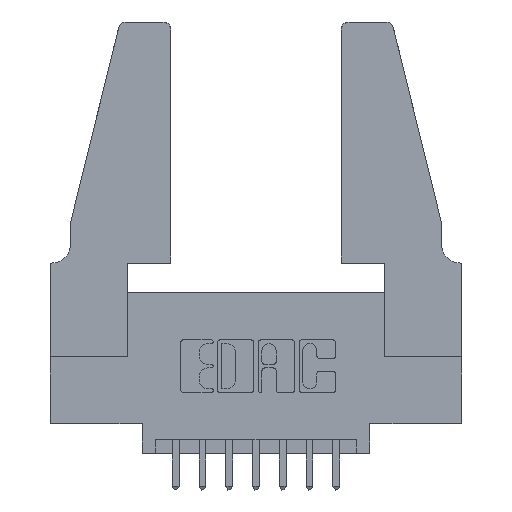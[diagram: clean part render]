
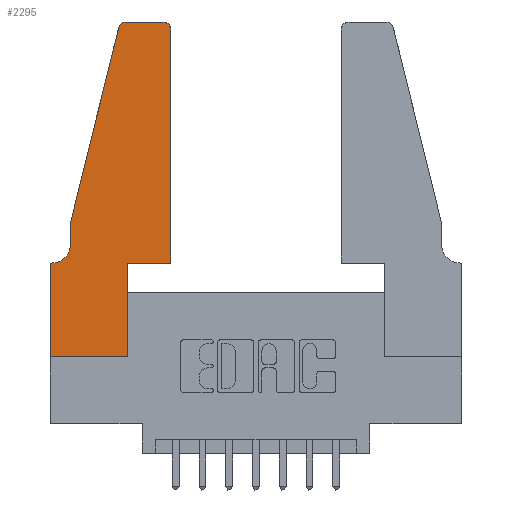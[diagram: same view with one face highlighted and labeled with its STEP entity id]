
A CAD part, top view. The second image highlights one B-rep face of the part: STEP entity #2295.
In plain terms, the highlighted planar face has unit normal (0, 0, 1).
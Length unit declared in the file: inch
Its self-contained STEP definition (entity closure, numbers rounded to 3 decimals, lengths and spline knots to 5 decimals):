
#74 = LINE ( 'NONE', #11500, #10061 ) ;
#209 = AXIS2_PLACEMENT_3D ( 'NONE', #2122, #8874, #3090 ) ;
#328 = CARTESIAN_POINT ( 'NONE',  ( 0.4505, 0.35, 0.37 ) ) ;
#382 = EDGE_CURVE ( 'NONE', #6844, #2311, #5477, .T. ) ;
#401 = VERTEX_POINT ( 'NONE', #3367 ) ;
#485 = CARTESIAN_POINT ( 'NONE',  ( 0.0755, 0.5, 0.37 ) ) ;
#541 = LINE ( 'NONE', #10446, #2849 ) ;
#887 = DIRECTION ( 'NONE',  ( 0., -1., 0. ) ) ;
#928 = EDGE_CURVE ( 'NONE', #4702, #10897, #2279, .T. ) ;
#1091 = DIRECTION ( 'NONE',  ( -0.239, -0.971, 0. ) ) ;
#1434 = EDGE_CURVE ( 'NONE', #10897, #5104, #6479, .T. ) ;
#1604 = VERTEX_POINT ( 'NONE', #1941 ) ;
#1919 = DIRECTION ( 'NONE',  ( 0., 1., 0. ) ) ;
#1941 = CARTESIAN_POINT ( 'NONE',  ( 0.2865, 0., 0.37 ) ) ;
#1979 = ORIENTED_EDGE ( 'NONE', *, *, #10025, .T. ) ;
#2013 = CARTESIAN_POINT ( 'NONE',  ( 0.0755, 0.42, 0.37 ) ) ;
#2122 = CARTESIAN_POINT ( 'NONE',  ( 0.0055, 0.42, 0.37 ) ) ;
#2279 = CIRCLE ( 'NONE', #3475, 0.03 ) ;
#2295 = ADVANCED_FACE ( 'NONE', ( #2711 ), #9443, .T. ) ;
#2311 = VERTEX_POINT ( 'NONE', #5641 ) ;
#2376 = EDGE_LOOP ( 'NONE', ( #1979, #10501, #11149, #3997, #9393, #7871, #9569, #4643, #2788, #7935, #9923, #3000 ) ) ;
#2415 = VECTOR ( 'NONE', #887, 39.37008 ) ;
#2492 = VERTEX_POINT ( 'NONE', #2013 ) ;
#2711 = FACE_OUTER_BOUND ( 'NONE', #2376, .T. ) ;
#2788 = ORIENTED_EDGE ( 'NONE', *, *, #5340, .T. ) ;
#2849 = VECTOR ( 'NONE', #3736, 39.37008 ) ;
#3000 = ORIENTED_EDGE ( 'NONE', *, *, #10651, .T. ) ;
#3090 = DIRECTION ( 'NONE',  ( -1., 0., 0. ) ) ;
#3192 = EDGE_CURVE ( 'NONE', #2311, #6945, #9752, .T. ) ;
#3367 = CARTESIAN_POINT ( 'NONE',  ( 0., 0., 0.37 ) ) ;
#3411 = CARTESIAN_POINT ( 'NONE',  ( 0.4505, 1.22, 0.37 ) ) ;
#3475 = AXIS2_PLACEMENT_3D ( 'NONE', #4786, #5442, #5460 ) ;
#3736 = DIRECTION ( 'NONE',  ( -1., 0., 0. ) ) ;
#3936 = VECTOR ( 'NONE', #1091, 39.37008 ) ;
#3997 = ORIENTED_EDGE ( 'NONE', *, *, #9315, .T. ) ;
#3998 = VECTOR ( 'NONE', #5031, 39.37008 ) ;
#4186 = LINE ( 'NONE', #8678, #9007 ) ;
#4343 = VERTEX_POINT ( 'NONE', #10725 ) ;
#4475 = DIRECTION ( 'NONE',  ( 1., 0., 0. ) ) ;
#4520 = LINE ( 'NONE', #11569, #9329 ) ;
#4643 = ORIENTED_EDGE ( 'NONE', *, *, #11556, .T. ) ;
#4702 = VERTEX_POINT ( 'NONE', #11522 ) ;
#4786 = CARTESIAN_POINT ( 'NONE',  ( 0.284, 1.22, 0.37 ) ) ;
#4874 = DIRECTION ( 'NONE',  ( -1., 0., 0. ) ) ;
#4983 = LINE ( 'NONE', #8634, #2415 ) ;
#5031 = DIRECTION ( 'NONE',  ( 1., 0., 0. ) ) ;
#5104 = VERTEX_POINT ( 'NONE', #9314 ) ;
#5340 = EDGE_CURVE ( 'NONE', #1604, #6844, #4186, .T. ) ;
#5442 = DIRECTION ( 'NONE',  ( 0., 0., 1. ) ) ;
#5460 = DIRECTION ( 'NONE',  ( 1., 0., 0. ) ) ;
#5477 = LINE ( 'NONE', #328, #10252 ) ;
#5494 = CARTESIAN_POINT ( 'NONE',  ( 0.4205, 1.22, 0.37 ) ) ;
#5641 = CARTESIAN_POINT ( 'NONE',  ( 0.4505, 0.35, 0.37 ) ) ;
#5959 = VERTEX_POINT ( 'NONE', #10536 ) ;
#5960 = CARTESIAN_POINT ( 'NONE',  ( 0., 0., 0.37 ) ) ;
#6087 = EDGE_CURVE ( 'NONE', #2492, #5959, #6267, .T. ) ;
#6267 = CIRCLE ( 'NONE', #209, 0.07 ) ;
#6432 = DIRECTION ( 'NONE',  ( 1., 0., 0. ) ) ;
#6479 = LINE ( 'NONE', #485, #3936 ) ;
#6728 = DIRECTION ( 'NONE',  ( 0., -1., 0. ) ) ;
#6844 = VERTEX_POINT ( 'NONE', #10929 ) ;
#6845 = LINE ( 'NONE', #5960, #3998 ) ;
#6945 = VERTEX_POINT ( 'NONE', #3411 ) ;
#7037 = CARTESIAN_POINT ( 'NONE',  ( 0.4505, 0.35, 0.37 ) ) ;
#7193 = VECTOR ( 'NONE', #12448, 39.37008 ) ;
#7871 = ORIENTED_EDGE ( 'NONE', *, *, #9899, .T. ) ;
#7935 = ORIENTED_EDGE ( 'NONE', *, *, #382, .T. ) ;
#8634 = CARTESIAN_POINT ( 'NONE',  ( 0.0755, 0.5, 0.37 ) ) ;
#8678 = CARTESIAN_POINT ( 'NONE',  ( 0.2865, 0.35, 0.37 ) ) ;
#8770 = VERTEX_POINT ( 'NONE', #9722 ) ;
#8874 = DIRECTION ( 'NONE',  ( 0., 0., -1. ) ) ;
#9007 = VECTOR ( 'NONE', #1919, 39.37008 ) ;
#9314 = CARTESIAN_POINT ( 'NONE',  ( 0.0755, 0.5, 0.37 ) ) ;
#9315 = EDGE_CURVE ( 'NONE', #5104, #2492, #4983, .T. ) ;
#9329 = VECTOR ( 'NONE', #4874, 39.37008 ) ;
#9393 = ORIENTED_EDGE ( 'NONE', *, *, #6087, .T. ) ;
#9443 = PLANE ( 'NONE',  #11101 ) ;
#9569 = ORIENTED_EDGE ( 'NONE', *, *, #10854, .T. ) ;
#9722 = CARTESIAN_POINT ( 'NONE',  ( 0.4205, 1.25, 0.37 ) ) ;
#9752 = LINE ( 'NONE', #7037, #7193 ) ;
#9899 = EDGE_CURVE ( 'NONE', #5959, #4343, #541, .T. ) ;
#9923 = ORIENTED_EDGE ( 'NONE', *, *, #3192, .T. ) ;
#10025 = EDGE_CURVE ( 'NONE', #8770, #4702, #4520, .T. ) ;
#10061 = VECTOR ( 'NONE', #6728, 39.37008 ) ;
#10252 = VECTOR ( 'NONE', #4475, 39.37008 ) ;
#10446 = CARTESIAN_POINT ( 'NONE',  ( 0.0755, 0.35, 0.37 ) ) ;
#10448 = AXIS2_PLACEMENT_3D ( 'NONE', #5494, #12182, #6432 ) ;
#10493 = DIRECTION ( 'NONE',  ( 0., 0., 1. ) ) ;
#10501 = ORIENTED_EDGE ( 'NONE', *, *, #928, .T. ) ;
#10536 = CARTESIAN_POINT ( 'NONE',  ( 0.0055, 0.35, 0.37 ) ) ;
#10651 = EDGE_CURVE ( 'NONE', #6945, #8770, #12486, .T. ) ;
#10690 = DIRECTION ( 'NONE',  ( 1., 0., 0. ) ) ;
#10725 = CARTESIAN_POINT ( 'NONE',  ( 0., 0.35, 0.37 ) ) ;
#10854 = EDGE_CURVE ( 'NONE', #4343, #401, #74, .T. ) ;
#10897 = VERTEX_POINT ( 'NONE', #11581 ) ;
#10929 = CARTESIAN_POINT ( 'NONE',  ( 0.2865, 0.35, 0.37 ) ) ;
#11101 = AXIS2_PLACEMENT_3D ( 'NONE', #11692, #10493, #10690 ) ;
#11149 = ORIENTED_EDGE ( 'NONE', *, *, #1434, .T. ) ;
#11500 = CARTESIAN_POINT ( 'NONE',  ( 0., 0., 0.37 ) ) ;
#11522 = CARTESIAN_POINT ( 'NONE',  ( 0.284, 1.25, 0.37 ) ) ;
#11556 = EDGE_CURVE ( 'NONE', #401, #1604, #6845, .T. ) ;
#11569 = CARTESIAN_POINT ( 'NONE',  ( 0.2605, 1.25, 0.37 ) ) ;
#11581 = CARTESIAN_POINT ( 'NONE',  ( 0.25487, 1.22718, 0.37 ) ) ;
#11692 = CARTESIAN_POINT ( 'NONE',  ( 0., 0.35, 0.37 ) ) ;
#12182 = DIRECTION ( 'NONE',  ( 0., 0., 1. ) ) ;
#12448 = DIRECTION ( 'NONE',  ( 0., 1., 0. ) ) ;
#12486 = CIRCLE ( 'NONE', #10448, 0.03 ) ;
